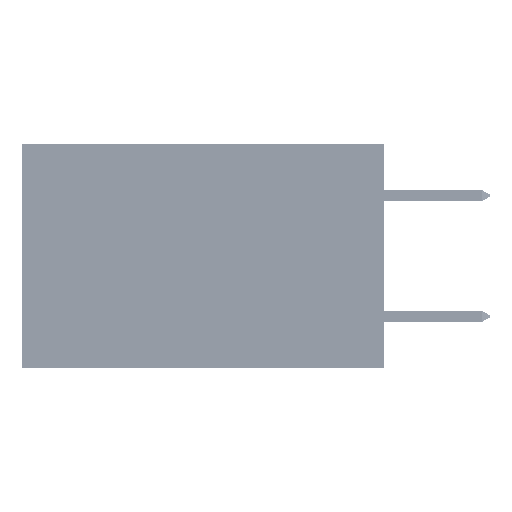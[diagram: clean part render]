
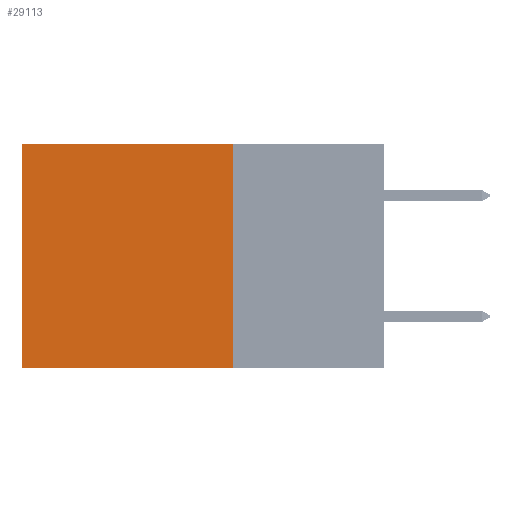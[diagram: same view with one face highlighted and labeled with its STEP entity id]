
A CAD part, left-side view. The second image highlights one B-rep face of the part: STEP entity #29113.
In plain terms, the highlighted planar face has unit normal (-1, 0, 0).
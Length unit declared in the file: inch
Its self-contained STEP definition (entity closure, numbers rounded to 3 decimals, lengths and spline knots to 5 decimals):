
#388 = CARTESIAN_POINT ( 'NONE',  ( 0.2875, 0.6, -0.37 ) ) ;
#942 = VERTEX_POINT ( 'NONE', #1397 ) ;
#1397 = CARTESIAN_POINT ( 'NONE',  ( 0.2875, 0.25, -0.37 ) ) ;
#3639 = VECTOR ( 'NONE', #10803, 39.37008 ) ;
#4181 = FACE_OUTER_BOUND ( 'NONE', #45512, .T. ) ;
#4425 = DIRECTION ( 'NONE',  ( 0., 0., -1. ) ) ;
#6381 = ORIENTED_EDGE ( 'NONE', *, *, #17158, .T. ) ;
#7523 = LINE ( 'NONE', #17648, #30307 ) ;
#8046 = LINE ( 'NONE', #46583, #36815 ) ;
#8939 = PLANE ( 'NONE',  #31967 ) ;
#10803 = DIRECTION ( 'NONE',  ( 0., 0., -1. ) ) ;
#12062 = DIRECTION ( 'NONE',  ( 0., 1., 0. ) ) ;
#12140 = ORIENTED_EDGE ( 'NONE', *, *, #29865, .F. ) ;
#13909 = EDGE_CURVE ( 'NONE', #40832, #942, #33107, .T. ) ;
#16240 = DIRECTION ( 'NONE',  ( 1., 0., 0. ) ) ;
#17158 = EDGE_CURVE ( 'NONE', #38575, #29093, #26898, .T. ) ;
#17648 = CARTESIAN_POINT ( 'NONE',  ( 0.2875, 0.25, 0. ) ) ;
#17733 = DIRECTION ( 'NONE',  ( 0., 0., -1. ) ) ;
#21284 = ORIENTED_EDGE ( 'NONE', *, *, #13909, .F. ) ;
#26898 = LINE ( 'NONE', #29926, #3639 ) ;
#28620 = EDGE_CURVE ( 'NONE', #40832, #38575, #7523, .T. ) ;
#29093 = VERTEX_POINT ( 'NONE', #388 ) ;
#29113 = ADVANCED_FACE ( 'NONE', ( #4181 ), #8939, .F. ) ;
#29865 = EDGE_CURVE ( 'NONE', #942, #29093, #8046, .T. ) ;
#29926 = CARTESIAN_POINT ( 'NONE',  ( 0.2875, 0.6, 0. ) ) ;
#30307 = VECTOR ( 'NONE', #48908, 39.37008 ) ;
#31967 = AXIS2_PLACEMENT_3D ( 'NONE', #42724, #16240, #4425 ) ;
#33107 = LINE ( 'NONE', #47748, #49303 ) ;
#36815 = VECTOR ( 'NONE', #12062, 39.37008 ) ;
#36838 = ORIENTED_EDGE ( 'NONE', *, *, #28620, .T. ) ;
#38575 = VERTEX_POINT ( 'NONE', #41709 ) ;
#40832 = VERTEX_POINT ( 'NONE', #48173 ) ;
#41709 = CARTESIAN_POINT ( 'NONE',  ( 0.2875, 0.6, 0. ) ) ;
#42724 = CARTESIAN_POINT ( 'NONE',  ( 0.2875, 0.25, 0. ) ) ;
#45512 = EDGE_LOOP ( 'NONE', ( #6381, #12140, #21284, #36838 ) ) ;
#46583 = CARTESIAN_POINT ( 'NONE',  ( 0.2875, 0.25, -0.37 ) ) ;
#47748 = CARTESIAN_POINT ( 'NONE',  ( 0.2875, 0.25, 0. ) ) ;
#48173 = CARTESIAN_POINT ( 'NONE',  ( 0.2875, 0.25, 0. ) ) ;
#48908 = DIRECTION ( 'NONE',  ( 0., 1., 0. ) ) ;
#49303 = VECTOR ( 'NONE', #17733, 39.37008 ) ;
